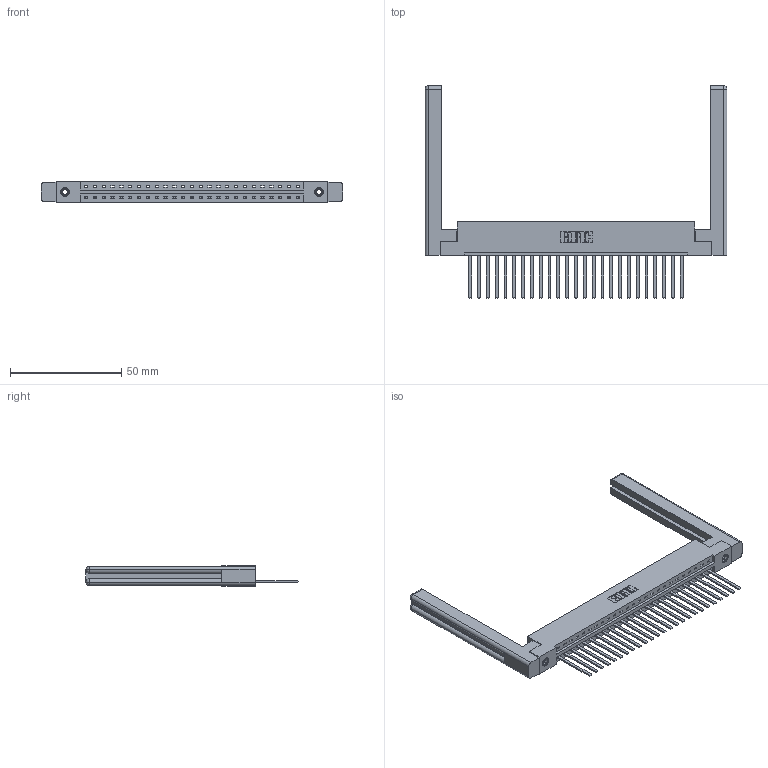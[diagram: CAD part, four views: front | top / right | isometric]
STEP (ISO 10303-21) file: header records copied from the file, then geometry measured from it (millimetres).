
FILE_DESCRIPTION (( 'STEP AP203' ), '1' );
FILE_NAME ('337-025-544-158.STEP', '2019-09-30T17:59:23', ( '' ), ( '' ), 'SwSTEP 2.0', 'SolidWorks 2016', '' );
FILE_SCHEMA (( 'CONFIG_CONTROL_DESIGN' ));
Length unit declared in the file: inch
Products named in the file (5): 337-025-544-158; 345-250-001_345-250-001-102; 345-292-001_345-293-144; 307-220-058; 337 Part_Flush Mounting Lugs - 0.156 Dia-TI
Assembly tree (30 placements, depth 2):
  337-025-544-158
    337 Part_Flush Mounting Lugs - 0.156 Dia-TI
    345-292-001_345-293-144  x25
    345-250-001_345-250-001-102  x2
    307-220-058  x2
Bounding box: 135.69 x 95.38 x 9.4 mm (x, y, z)
Volume: 21341.3 mm3; surface area: 20723.2 mm2
Topology: 30 solids, 30 shells, 1656 faces, 4915 edges, 3230 vertices
Faces by surface type: plane 1204, cylinder 428, cone 12, torus 12
Entity records: 23232 total; most frequent: CARTESIAN_POINT 4044, ORIENTED_EDGE 3944, DIRECTION 3454, EDGE_CURVE 1972, LINE 1800, VECTOR 1800, VERTEX_POINT 1306, AXIS2_PLACEMENT_3D 827
